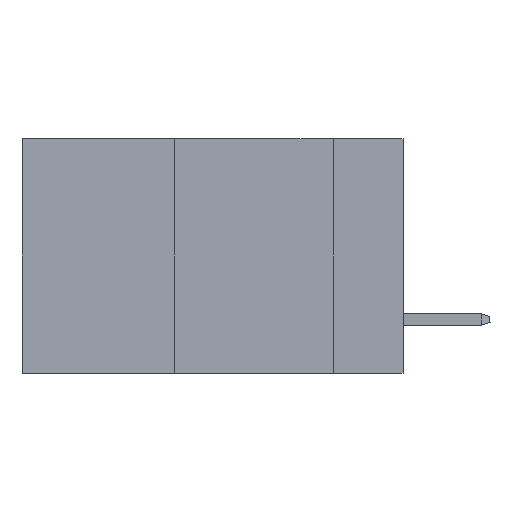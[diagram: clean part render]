
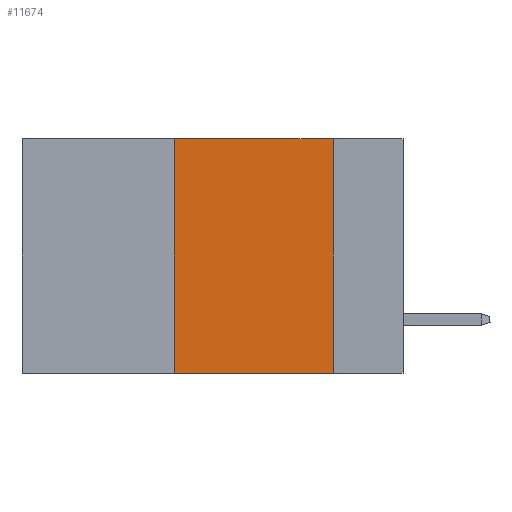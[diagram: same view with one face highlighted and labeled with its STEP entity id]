
A CAD part, left-side view. The second image highlights one B-rep face of the part: STEP entity #11674.
In plain terms, the highlighted planar face has unit normal (-1, 0, 0).
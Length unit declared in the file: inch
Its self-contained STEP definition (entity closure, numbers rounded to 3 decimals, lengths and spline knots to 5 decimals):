
#1087 = DIRECTION ( 'NONE',  ( 1., 0., 0. ) ) ;
#1202 = VECTOR ( 'NONE', #8004, 39.37008 ) ;
#2607 = PLANE ( 'NONE',  #5385 ) ;
#3317 = VECTOR ( 'NONE', #9419, 39.37008 ) ;
#3445 = CARTESIAN_POINT ( 'NONE',  ( 0., 0.6, -0.37 ) ) ;
#4124 = CARTESIAN_POINT ( 'NONE',  ( 0., 0.11, 0. ) ) ;
#4458 = VERTEX_POINT ( 'NONE', #7987 ) ;
#5282 = CARTESIAN_POINT ( 'NONE',  ( 0., 0.36, 0. ) ) ;
#5385 = AXIS2_PLACEMENT_3D ( 'NONE', #8994, #1087, #14215 ) ;
#5411 = LINE ( 'NONE', #4124, #3317 ) ;
#5672 = EDGE_CURVE ( 'NONE', #4458, #16010, #5411, .T. ) ;
#6514 = VERTEX_POINT ( 'NONE', #16206 ) ;
#6649 = DIRECTION ( 'NONE',  ( 0., -1., 0. ) ) ;
#6820 = LINE ( 'NONE', #9535, #14797 ) ;
#7438 = ORIENTED_EDGE ( 'NONE', *, *, #5672, .F. ) ;
#7628 = FACE_OUTER_BOUND ( 'NONE', #11346, .T. ) ;
#7971 = EDGE_CURVE ( 'NONE', #6514, #16010, #9859, .T. ) ;
#7987 = CARTESIAN_POINT ( 'NONE',  ( 0., 0.11, 0. ) ) ;
#8004 = DIRECTION ( 'NONE',  ( 0., 0., 1. ) ) ;
#8547 = DIRECTION ( 'NONE',  ( 0., -1., 0. ) ) ;
#8938 = ORIENTED_EDGE ( 'NONE', *, *, #7971, .T. ) ;
#8994 = CARTESIAN_POINT ( 'NONE',  ( 0., 0.6, 0. ) ) ;
#9419 = DIRECTION ( 'NONE',  ( 0., 0., -1. ) ) ;
#9484 = LINE ( 'NONE', #10761, #1202 ) ;
#9535 = CARTESIAN_POINT ( 'NONE',  ( 0., 0.6, 0. ) ) ;
#9553 = EDGE_CURVE ( 'NONE', #6514, #12209, #9484, .T. ) ;
#9859 = LINE ( 'NONE', #3445, #15683 ) ;
#10761 = CARTESIAN_POINT ( 'NONE',  ( 0., 0.36, 0. ) ) ;
#11346 = EDGE_LOOP ( 'NONE', ( #7438, #12873, #13183, #8938 ) ) ;
#11674 = ADVANCED_FACE ( 'NONE', ( #7628 ), #2607, .F. ) ;
#12209 = VERTEX_POINT ( 'NONE', #5282 ) ;
#12430 = EDGE_CURVE ( 'NONE', #12209, #4458, #6820, .T. ) ;
#12873 = ORIENTED_EDGE ( 'NONE', *, *, #12430, .F. ) ;
#13183 = ORIENTED_EDGE ( 'NONE', *, *, #9553, .F. ) ;
#14215 = DIRECTION ( 'NONE',  ( 0., 0., -1. ) ) ;
#14715 = CARTESIAN_POINT ( 'NONE',  ( 0., 0.11, -0.37 ) ) ;
#14797 = VECTOR ( 'NONE', #6649, 39.37008 ) ;
#15683 = VECTOR ( 'NONE', #8547, 39.37008 ) ;
#16010 = VERTEX_POINT ( 'NONE', #14715 ) ;
#16206 = CARTESIAN_POINT ( 'NONE',  ( 0., 0.36, -0.37 ) ) ;
